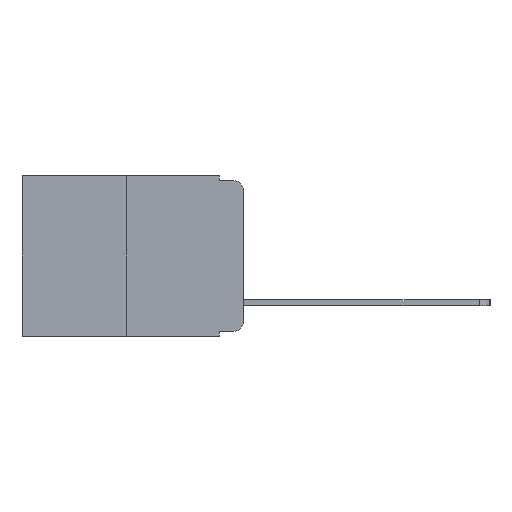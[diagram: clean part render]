
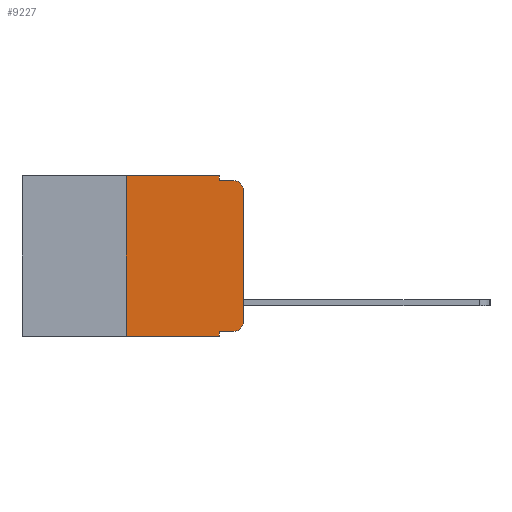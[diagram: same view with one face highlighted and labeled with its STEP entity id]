
A CAD part, left-side view. The second image highlights one B-rep face of the part: STEP entity #9227.
In plain terms, the highlighted planar face has unit normal (-1, 0, 0).
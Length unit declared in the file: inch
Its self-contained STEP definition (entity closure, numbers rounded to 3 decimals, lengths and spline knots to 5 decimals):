
#98 = DIRECTION ( 'NONE',  ( 0., -1., 0. ) ) ;
#283 = DIRECTION ( 'NONE',  ( 0., -1., 0. ) ) ;
#413 = ORIENTED_EDGE ( 'NONE', *, *, #966, .T. ) ;
#908 = CARTESIAN_POINT ( 'NONE',  ( 0., 0., -0.313 ) ) ;
#966 = EDGE_CURVE ( 'NONE', #8217, #3539, #15540, .T. ) ;
#1373 = ORIENTED_EDGE ( 'NONE', *, *, #9315, .F. ) ;
#1599 = CARTESIAN_POINT ( 'NONE',  ( 0., 0.051, 0. ) ) ;
#1737 = FACE_OUTER_BOUND ( 'NONE', #21163, .T. ) ;
#2255 = ORIENTED_EDGE ( 'NONE', *, *, #12566, .T. ) ;
#2500 = CARTESIAN_POINT ( 'NONE',  ( 0., 0.02, -0.333 ) ) ;
#2883 = ORIENTED_EDGE ( 'NONE', *, *, #4562, .T. ) ;
#2984 = VECTOR ( 'NONE', #15872, 39.37008 ) ;
#3334 = CARTESIAN_POINT ( 'NONE',  ( 0., 0.02, -0.03 ) ) ;
#3470 = CARTESIAN_POINT ( 'NONE',  ( 0., 0.473, 0. ) ) ;
#3539 = VERTEX_POINT ( 'NONE', #908 ) ;
#3651 = ORIENTED_EDGE ( 'NONE', *, *, #16768, .T. ) ;
#3946 = VERTEX_POINT ( 'NONE', #18974 ) ;
#4039 = CARTESIAN_POINT ( 'NONE',  ( 0., 0.25, 0. ) ) ;
#4203 = VERTEX_POINT ( 'NONE', #5005 ) ;
#4562 = EDGE_CURVE ( 'NONE', #8139, #8217, #6880, .T. ) ;
#4946 = LINE ( 'NONE', #19900, #13422 ) ;
#5005 = CARTESIAN_POINT ( 'NONE',  ( 0., 0.051, -0.343 ) ) ;
#5119 = DIRECTION ( 'NONE',  ( 0., 0., -1. ) ) ;
#5148 = ORIENTED_EDGE ( 'NONE', *, *, #11447, .F. ) ;
#5259 = VECTOR ( 'NONE', #11662, 39.37008 ) ;
#5271 = DIRECTION ( 'NONE',  ( 0., 0., -1. ) ) ;
#5706 = EDGE_CURVE ( 'NONE', #8139, #4203, #12207, .T. ) ;
#6354 = ORIENTED_EDGE ( 'NONE', *, *, #5706, .F. ) ;
#6469 = CARTESIAN_POINT ( 'NONE',  ( 0., 0.02, -0.313 ) ) ;
#6489 = DIRECTION ( 'NONE',  ( -1., 0., 0. ) ) ;
#6835 = EDGE_CURVE ( 'NONE', #21344, #19954, #7062, .T. ) ;
#6880 = LINE ( 'NONE', #7736, #15325 ) ;
#6967 = ORIENTED_EDGE ( 'NONE', *, *, #8007, .F. ) ;
#7062 = LINE ( 'NONE', #4039, #2984 ) ;
#7111 = AXIS2_PLACEMENT_3D ( 'NONE', #6469, #6489, #13161 ) ;
#7163 = CARTESIAN_POINT ( 'NONE',  ( 0., 0.25, -0.343 ) ) ;
#7736 = CARTESIAN_POINT ( 'NONE',  ( 0., 0.051, -0.333 ) ) ;
#8007 = EDGE_CURVE ( 'NONE', #8743, #3946, #20884, .T. ) ;
#8139 = VERTEX_POINT ( 'NONE', #15948 ) ;
#8217 = VERTEX_POINT ( 'NONE', #2500 ) ;
#8370 = VERTEX_POINT ( 'NONE', #9812 ) ;
#8743 = VERTEX_POINT ( 'NONE', #21395 ) ;
#8903 = CARTESIAN_POINT ( 'NONE',  ( 0., 0.051, 0. ) ) ;
#9227 = ADVANCED_FACE ( 'NONE', ( #1737 ), #13690, .F. ) ;
#9315 = EDGE_CURVE ( 'NONE', #19954, #8743, #21099, .T. ) ;
#9812 = CARTESIAN_POINT ( 'NONE',  ( 0., 0.02, -0.01 ) ) ;
#10290 = DIRECTION ( 'NONE',  ( 0., -1., 0. ) ) ;
#10300 = LINE ( 'NONE', #13242, #5259 ) ;
#10587 = CARTESIAN_POINT ( 'NONE',  ( 0., 0.473, -0.343 ) ) ;
#10671 = AXIS2_PLACEMENT_3D ( 'NONE', #3470, #15358, #5271 ) ;
#10685 = CARTESIAN_POINT ( 'NONE',  ( 0., 0.473, 0. ) ) ;
#10828 = VECTOR ( 'NONE', #98, 39.37008 ) ;
#11447 = EDGE_CURVE ( 'NONE', #3946, #8370, #4946, .T. ) ;
#11460 = ORIENTED_EDGE ( 'NONE', *, *, #6835, .F. ) ;
#11662 = DIRECTION ( 'NONE',  ( 0., 0., 1. ) ) ;
#12207 = LINE ( 'NONE', #1599, #20074 ) ;
#12566 = EDGE_CURVE ( 'NONE', #13588, #8370, #18576, .T. ) ;
#13161 = DIRECTION ( 'NONE',  ( 0., 0., -1. ) ) ;
#13242 = CARTESIAN_POINT ( 'NONE',  ( 0., 0., 0. ) ) ;
#13422 = VECTOR ( 'NONE', #10290, 39.37008 ) ;
#13556 = AXIS2_PLACEMENT_3D ( 'NONE', #3334, #15214, #5119 ) ;
#13588 = VERTEX_POINT ( 'NONE', #20881 ) ;
#13649 = EDGE_CURVE ( 'NONE', #3539, #13588, #10300, .T. ) ;
#13690 = PLANE ( 'NONE',  #10671 ) ;
#13815 = VECTOR ( 'NONE', #283, 39.37008 ) ;
#14216 = CARTESIAN_POINT ( 'NONE',  ( 0., 0.25, 0. ) ) ;
#15214 = DIRECTION ( 'NONE',  ( -1., 0., 0. ) ) ;
#15325 = VECTOR ( 'NONE', #16071, 39.37008 ) ;
#15358 = DIRECTION ( 'NONE',  ( 1., 0., 0. ) ) ;
#15540 = CIRCLE ( 'NONE', #7111, 0.02 ) ;
#15872 = DIRECTION ( 'NONE',  ( 0., 0., 1. ) ) ;
#15948 = CARTESIAN_POINT ( 'NONE',  ( 0., 0.051, -0.333 ) ) ;
#16071 = DIRECTION ( 'NONE',  ( 0., -1., 0. ) ) ;
#16336 = ORIENTED_EDGE ( 'NONE', *, *, #13649, .T. ) ;
#16768 = EDGE_CURVE ( 'NONE', #21344, #4203, #19354, .T. ) ;
#18576 = CIRCLE ( 'NONE', #13556, 0.02 ) ;
#18974 = CARTESIAN_POINT ( 'NONE',  ( 0., 0.051, -0.01 ) ) ;
#19354 = LINE ( 'NONE', #10587, #10828 ) ;
#19900 = CARTESIAN_POINT ( 'NONE',  ( 0., 0.051, -0.01 ) ) ;
#19954 = VERTEX_POINT ( 'NONE', #14216 ) ;
#20074 = VECTOR ( 'NONE', #21351, 39.37008 ) ;
#20204 = DIRECTION ( 'NONE',  ( 0., 0., -1. ) ) ;
#20407 = VECTOR ( 'NONE', #20204, 39.37008 ) ;
#20881 = CARTESIAN_POINT ( 'NONE',  ( 0., 0., -0.03 ) ) ;
#20884 = LINE ( 'NONE', #8903, #20407 ) ;
#21099 = LINE ( 'NONE', #10685, #13815 ) ;
#21163 = EDGE_LOOP ( 'NONE', ( #16336, #2255, #5148, #6967, #1373, #11460, #3651, #6354, #2883, #413 ) ) ;
#21344 = VERTEX_POINT ( 'NONE', #7163 ) ;
#21351 = DIRECTION ( 'NONE',  ( 0., 0., -1. ) ) ;
#21395 = CARTESIAN_POINT ( 'NONE',  ( 0., 0.051, 0. ) ) ;
